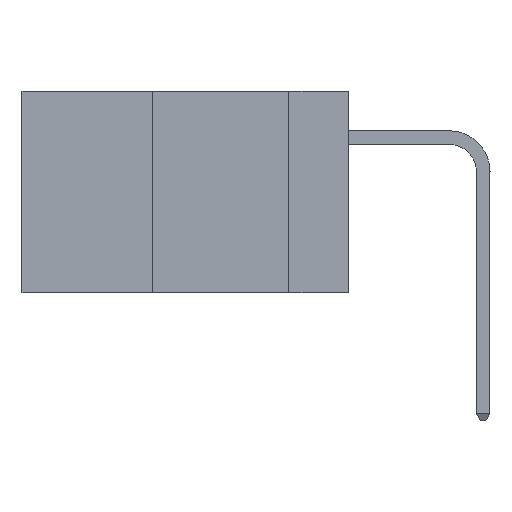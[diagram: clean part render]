
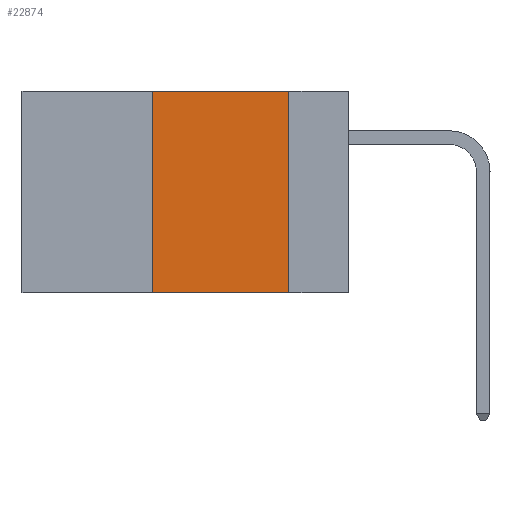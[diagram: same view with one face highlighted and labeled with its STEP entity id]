
A CAD part, left-side view. The second image highlights one B-rep face of the part: STEP entity #22874.
In plain terms, the highlighted planar face has unit normal (-1, 0, 0).
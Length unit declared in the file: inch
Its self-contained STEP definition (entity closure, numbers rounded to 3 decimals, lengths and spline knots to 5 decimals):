
#255 = CARTESIAN_POINT ( 'NONE',  ( 0., 0.36, 0. ) ) ;
#472 = LINE ( 'NONE', #3614, #22910 ) ;
#499 = ORIENTED_EDGE ( 'NONE', *, *, #14521, .T. ) ;
#1163 = EDGE_CURVE ( 'NONE', #23543, #19659, #6353, .T. ) ;
#3533 = EDGE_LOOP ( 'NONE', ( #5163, #20967, #6771, #499 ) ) ;
#3614 = CARTESIAN_POINT ( 'NONE',  ( 0., 0.36, 0. ) ) ;
#3878 = CARTESIAN_POINT ( 'NONE',  ( 0., 0.11, 0. ) ) ;
#4766 = FACE_OUTER_BOUND ( 'NONE', #3533, .T. ) ;
#5063 = DIRECTION ( 'NONE',  ( 0., 0., -1. ) ) ;
#5163 = ORIENTED_EDGE ( 'NONE', *, *, #20776, .F. ) ;
#5406 = EDGE_CURVE ( 'NONE', #8224, #23543, #472, .T. ) ;
#6353 = LINE ( 'NONE', #6612, #27233 ) ;
#6612 = CARTESIAN_POINT ( 'NONE',  ( 0., 0.6, 0. ) ) ;
#6771 = ORIENTED_EDGE ( 'NONE', *, *, #5406, .F. ) ;
#6985 = LINE ( 'NONE', #11635, #16460 ) ;
#8224 = VERTEX_POINT ( 'NONE', #14209 ) ;
#11115 = DIRECTION ( 'NONE',  ( 1., 0., 0. ) ) ;
#11635 = CARTESIAN_POINT ( 'NONE',  ( 0., 0.11, 0. ) ) ;
#13539 = VERTEX_POINT ( 'NONE', #19717 ) ;
#13600 = DIRECTION ( 'NONE',  ( 0., 0., 1. ) ) ;
#13728 = DIRECTION ( 'NONE',  ( 0., -1., 0. ) ) ;
#14209 = CARTESIAN_POINT ( 'NONE',  ( 0., 0.36, -0.37 ) ) ;
#14521 = EDGE_CURVE ( 'NONE', #8224, #13539, #14764, .T. ) ;
#14610 = AXIS2_PLACEMENT_3D ( 'NONE', #17536, #11115, #26130 ) ;
#14764 = LINE ( 'NONE', #27158, #20443 ) ;
#16460 = VECTOR ( 'NONE', #5063, 39.37008 ) ;
#17536 = CARTESIAN_POINT ( 'NONE',  ( 0., 0.6, 0. ) ) ;
#18635 = DIRECTION ( 'NONE',  ( 0., -1., 0. ) ) ;
#19659 = VERTEX_POINT ( 'NONE', #3878 ) ;
#19717 = CARTESIAN_POINT ( 'NONE',  ( 0., 0.11, -0.37 ) ) ;
#20443 = VECTOR ( 'NONE', #18635, 39.37008 ) ;
#20776 = EDGE_CURVE ( 'NONE', #19659, #13539, #6985, .T. ) ;
#20967 = ORIENTED_EDGE ( 'NONE', *, *, #1163, .F. ) ;
#22874 = ADVANCED_FACE ( 'NONE', ( #4766 ), #23935, .F. ) ;
#22910 = VECTOR ( 'NONE', #13600, 39.37008 ) ;
#23543 = VERTEX_POINT ( 'NONE', #255 ) ;
#23935 = PLANE ( 'NONE',  #14610 ) ;
#26130 = DIRECTION ( 'NONE',  ( 0., 0., -1. ) ) ;
#27158 = CARTESIAN_POINT ( 'NONE',  ( 0., 0.6, -0.37 ) ) ;
#27233 = VECTOR ( 'NONE', #13728, 39.37008 ) ;
